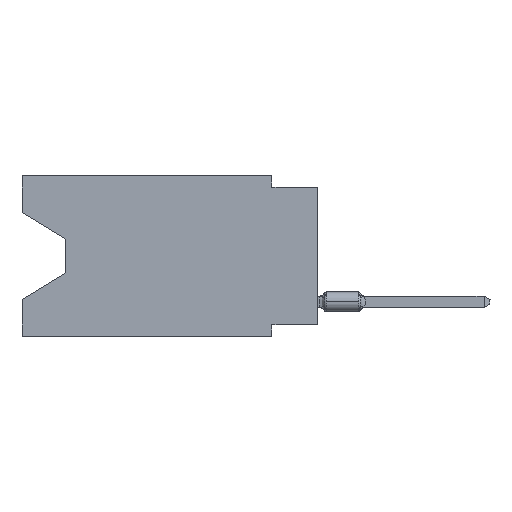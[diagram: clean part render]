
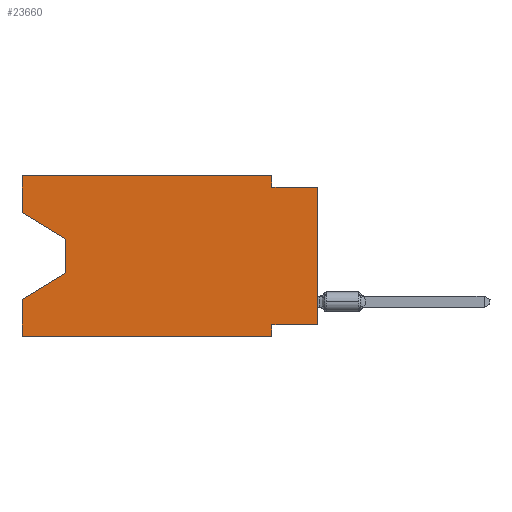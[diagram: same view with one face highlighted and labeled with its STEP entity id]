
A CAD part, left-side view. The second image highlights one B-rep face of the part: STEP entity #23660.
In plain terms, the highlighted planar face has unit normal (-1, 0, 0).
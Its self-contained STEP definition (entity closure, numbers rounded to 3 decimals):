
#159 = DIRECTION ( 'NONE',  ( 0., 0., 1. ) ) ;
#643 = CARTESIAN_POINT ( 'NONE',  ( 0., 16.383, -8.89 ) ) ;
#998 = DIRECTION ( 'NONE',  ( 0., 0., -1. ) ) ;
#1286 = VECTOR ( 'NONE', #32573, 1000. ) ;
#1799 = CARTESIAN_POINT ( 'NONE',  ( 0., 13.97, -3.505 ) ) ;
#2451 = CARTESIAN_POINT ( 'NONE',  ( 0., 16.383, -6.852 ) ) ;
#3424 = CARTESIAN_POINT ( 'NONE',  ( 0., 13.97, -5.385 ) ) ;
#3710 = CARTESIAN_POINT ( 'NONE',  ( 0., 2.54, -8.89 ) ) ;
#4681 = CARTESIAN_POINT ( 'NONE',  ( 0., 0., -0.635 ) ) ;
#4933 = LINE ( 'NONE', #50726, #7830 ) ;
#6979 = LINE ( 'NONE', #10572, #13007 ) ;
#7431 = VECTOR ( 'NONE', #43555, 1000. ) ;
#7653 = ORIENTED_EDGE ( 'NONE', *, *, #47926, .T. ) ;
#7830 = VECTOR ( 'NONE', #19497, 1000. ) ;
#8461 = ORIENTED_EDGE ( 'NONE', *, *, #13586, .T. ) ;
#8630 = EDGE_CURVE ( 'NONE', #19508, #57657, #48260, .T. ) ;
#9356 = ORIENTED_EDGE ( 'NONE', *, *, #15934, .F. ) ;
#10239 = LINE ( 'NONE', #56853, #51956 ) ;
#10342 = EDGE_CURVE ( 'NONE', #57657, #45124, #13778, .T. ) ;
#10572 = CARTESIAN_POINT ( 'NONE',  ( 0., 0., -8.255 ) ) ;
#11558 = LINE ( 'NONE', #1799, #25261 ) ;
#11949 = CARTESIAN_POINT ( 'NONE',  ( 0., 2.54, 0. ) ) ;
#12261 = ORIENTED_EDGE ( 'NONE', *, *, #14879, .F. ) ;
#13007 = VECTOR ( 'NONE', #43239, 1000. ) ;
#13225 = EDGE_CURVE ( 'NONE', #31893, #15599, #23316, .T. ) ;
#13586 = EDGE_CURVE ( 'NONE', #31270, #58450, #26812, .T. ) ;
#13778 = LINE ( 'NONE', #18834, #15512 ) ;
#14879 = EDGE_CURVE ( 'NONE', #45124, #15599, #10239, .T. ) ;
#15512 = VECTOR ( 'NONE', #998, 1000. ) ;
#15599 = VERTEX_POINT ( 'NONE', #4681 ) ;
#15934 = EDGE_CURVE ( 'NONE', #18806, #46127, #31033, .T. ) ;
#16231 = LINE ( 'NONE', #38258, #33528 ) ;
#18806 = VERTEX_POINT ( 'NONE', #24211 ) ;
#18834 = CARTESIAN_POINT ( 'NONE',  ( 0., 2.54, 0. ) ) ;
#19497 = DIRECTION ( 'NONE',  ( 0., 0., 1. ) ) ;
#19508 = VERTEX_POINT ( 'NONE', #49294 ) ;
#20418 = DIRECTION ( 'NONE',  ( 0., 0., 1. ) ) ;
#22910 = VECTOR ( 'NONE', #40196, 1000. ) ;
#23077 = CARTESIAN_POINT ( 'NONE',  ( 0., 2.54, -0.635 ) ) ;
#23316 = LINE ( 'NONE', #40882, #44396 ) ;
#23660 = ADVANCED_FACE ( 'NONE', ( #36485 ), #32582, .F. ) ;
#24211 = CARTESIAN_POINT ( 'NONE',  ( 0., 2.54, -8.255 ) ) ;
#25261 = VECTOR ( 'NONE', #38333, 1000. ) ;
#26812 = LINE ( 'NONE', #58653, #32067 ) ;
#27564 = ORIENTED_EDGE ( 'NONE', *, *, #10342, .F. ) ;
#27878 = ORIENTED_EDGE ( 'NONE', *, *, #50185, .F. ) ;
#29326 = ORIENTED_EDGE ( 'NONE', *, *, #55252, .T. ) ;
#29684 = DIRECTION ( 'NONE',  ( 0., -1., 0. ) ) ;
#30664 = CARTESIAN_POINT ( 'NONE',  ( 0., 16.383, 0. ) ) ;
#31033 = LINE ( 'NONE', #3710, #7431 ) ;
#31270 = VERTEX_POINT ( 'NONE', #3424 ) ;
#31612 = VERTEX_POINT ( 'NONE', #50281 ) ;
#31803 = EDGE_CURVE ( 'NONE', #34907, #46127, #34164, .T. ) ;
#31893 = VERTEX_POINT ( 'NONE', #47565 ) ;
#32009 = DIRECTION ( 'NONE',  ( 1., 0., 0. ) ) ;
#32067 = VECTOR ( 'NONE', #44980, 1000. ) ;
#32083 = ORIENTED_EDGE ( 'NONE', *, *, #13225, .T. ) ;
#32573 = DIRECTION ( 'NONE',  ( 0., -0.855, -0.519 ) ) ;
#32582 = PLANE ( 'NONE',  #44143 ) ;
#33179 = LINE ( 'NONE', #46001, #1286 ) ;
#33528 = VECTOR ( 'NONE', #20418, 1000. ) ;
#34164 = LINE ( 'NONE', #51172, #45873 ) ;
#34907 = VERTEX_POINT ( 'NONE', #643 ) ;
#36485 = FACE_OUTER_BOUND ( 'NONE', #40874, .T. ) ;
#37061 = ORIENTED_EDGE ( 'NONE', *, *, #57169, .F. ) ;
#38258 = CARTESIAN_POINT ( 'NONE',  ( 0., 16.383, 0. ) ) ;
#38333 = DIRECTION ( 'NONE',  ( 0., 0., -1. ) ) ;
#40196 = DIRECTION ( 'NONE',  ( 0., -1., 0. ) ) ;
#40874 = EDGE_LOOP ( 'NONE', ( #29326, #7653, #8461, #37061, #43678, #9356, #52508, #32083, #12261, #27564, #56045, #27878 ) ) ;
#40882 = CARTESIAN_POINT ( 'NONE',  ( 0., 0., 0. ) ) ;
#41830 = CARTESIAN_POINT ( 'NONE',  ( 0., 16.383, 0. ) ) ;
#43239 = DIRECTION ( 'NONE',  ( 0., 1., 0. ) ) ;
#43555 = DIRECTION ( 'NONE',  ( 0., 0., -1. ) ) ;
#43678 = ORIENTED_EDGE ( 'NONE', *, *, #31803, .T. ) ;
#44143 = AXIS2_PLACEMENT_3D ( 'NONE', #41830, #32009, #54029 ) ;
#44396 = VECTOR ( 'NONE', #159, 1000. ) ;
#44980 = DIRECTION ( 'NONE',  ( 0., 0.855, -0.519 ) ) ;
#45124 = VERTEX_POINT ( 'NONE', #23077 ) ;
#45873 = VECTOR ( 'NONE', #29684, 1000. ) ;
#46001 = CARTESIAN_POINT ( 'NONE',  ( 0., 16.383, -2.038 ) ) ;
#46127 = VERTEX_POINT ( 'NONE', #57903 ) ;
#46178 = CARTESIAN_POINT ( 'NONE',  ( 0., 16.383, -2.038 ) ) ;
#47565 = CARTESIAN_POINT ( 'NONE',  ( 0., 0., -8.255 ) ) ;
#47926 = EDGE_CURVE ( 'NONE', #31612, #31270, #11558, .T. ) ;
#48260 = LINE ( 'NONE', #30664, #22910 ) ;
#48824 = EDGE_CURVE ( 'NONE', #31893, #18806, #6979, .T. ) ;
#49294 = CARTESIAN_POINT ( 'NONE',  ( 0., 16.383, 0. ) ) ;
#50185 = EDGE_CURVE ( 'NONE', #58364, #19508, #16231, .T. ) ;
#50281 = CARTESIAN_POINT ( 'NONE',  ( 0., 13.97, -3.505 ) ) ;
#50726 = CARTESIAN_POINT ( 'NONE',  ( 0., 16.383, 0. ) ) ;
#51172 = CARTESIAN_POINT ( 'NONE',  ( 0., 16.383, -8.89 ) ) ;
#51512 = DIRECTION ( 'NONE',  ( 0., -1., 0. ) ) ;
#51956 = VECTOR ( 'NONE', #51512, 1000. ) ;
#52508 = ORIENTED_EDGE ( 'NONE', *, *, #48824, .F. ) ;
#54029 = DIRECTION ( 'NONE',  ( 0., 0., -1. ) ) ;
#55252 = EDGE_CURVE ( 'NONE', #58364, #31612, #33179, .T. ) ;
#56045 = ORIENTED_EDGE ( 'NONE', *, *, #8630, .F. ) ;
#56853 = CARTESIAN_POINT ( 'NONE',  ( 0., 0., -0.635 ) ) ;
#57169 = EDGE_CURVE ( 'NONE', #34907, #58450, #4933, .T. ) ;
#57657 = VERTEX_POINT ( 'NONE', #11949 ) ;
#57903 = CARTESIAN_POINT ( 'NONE',  ( 0., 2.54, -8.89 ) ) ;
#58364 = VERTEX_POINT ( 'NONE', #46178 ) ;
#58450 = VERTEX_POINT ( 'NONE', #2451 ) ;
#58653 = CARTESIAN_POINT ( 'NONE',  ( 0., 13.97, -5.385 ) ) ;
